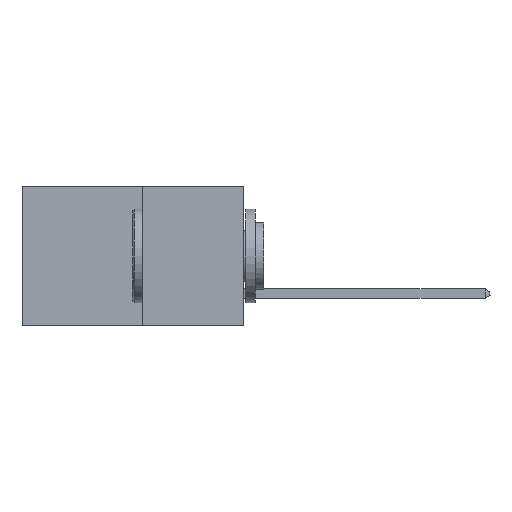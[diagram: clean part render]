
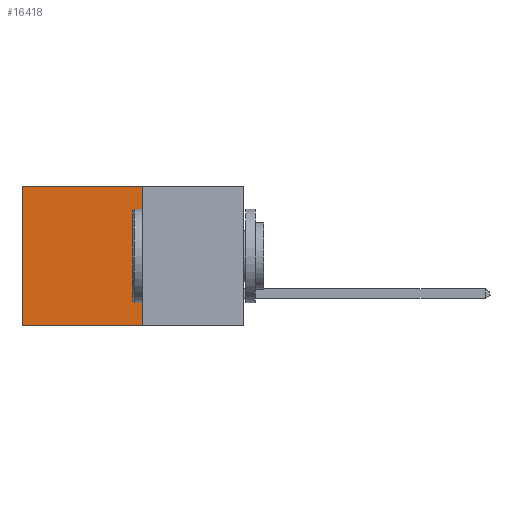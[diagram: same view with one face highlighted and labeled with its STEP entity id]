
A CAD part, left-side view. The second image highlights one B-rep face of the part: STEP entity #16418.
In plain terms, the highlighted planar face has unit normal (-1, 0, 0).
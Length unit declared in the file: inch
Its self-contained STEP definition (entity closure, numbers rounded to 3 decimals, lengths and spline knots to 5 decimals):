
#1302 = EDGE_CURVE ( 'NONE', #14299, #14723, #8624, .T. ) ;
#1588 = VECTOR ( 'NONE', #5379, 39.37008 ) ;
#3808 = LINE ( 'NONE', #8963, #6891 ) ;
#4019 = EDGE_CURVE ( 'NONE', #6749, #14299, #8318, .T. ) ;
#4483 = AXIS2_PLACEMENT_3D ( 'NONE', #4755, #16290, #8631 ) ;
#4755 = CARTESIAN_POINT ( 'NONE',  ( 0.277, 0.27, -0.37 ) ) ;
#4781 = CARTESIAN_POINT ( 'NONE',  ( 0.277, 0.27, -0.37 ) ) ;
#4987 = CARTESIAN_POINT ( 'NONE',  ( 0.277, 0.27, 0. ) ) ;
#5379 = DIRECTION ( 'NONE',  ( 0., 0., -1. ) ) ;
#5942 = VERTEX_POINT ( 'NONE', #13250 ) ;
#6466 = ORIENTED_EDGE ( 'NONE', *, *, #4019, .F. ) ;
#6491 = CARTESIAN_POINT ( 'NONE',  ( 0.277, 0.59, -0.37 ) ) ;
#6749 = VERTEX_POINT ( 'NONE', #11069 ) ;
#6891 = VECTOR ( 'NONE', #16617, 39.37008 ) ;
#7276 = DIRECTION ( 'NONE',  ( 0., 1., 0. ) ) ;
#7335 = PLANE ( 'NONE',  #4483 ) ;
#7648 = FACE_OUTER_BOUND ( 'NONE', #14493, .T. ) ;
#7660 = EDGE_CURVE ( 'NONE', #5942, #14723, #3808, .T. ) ;
#7832 = VECTOR ( 'NONE', #7276, 39.37008 ) ;
#8318 = LINE ( 'NONE', #4781, #1588 ) ;
#8624 = LINE ( 'NONE', #10441, #7832 ) ;
#8631 = DIRECTION ( 'NONE',  ( 0., 0., -1. ) ) ;
#8956 = VECTOR ( 'NONE', #10148, 39.37008 ) ;
#8963 = CARTESIAN_POINT ( 'NONE',  ( 0.277, 0.59, -0.37 ) ) ;
#10148 = DIRECTION ( 'NONE',  ( 0., 1., 0. ) ) ;
#10441 = CARTESIAN_POINT ( 'NONE',  ( 0.277, 0.27, -0.37 ) ) ;
#11069 = CARTESIAN_POINT ( 'NONE',  ( 0.277, 0.27, 0. ) ) ;
#11328 = EDGE_CURVE ( 'NONE', #6749, #5942, #15789, .T. ) ;
#11894 = ORIENTED_EDGE ( 'NONE', *, *, #1302, .F. ) ;
#13238 = CARTESIAN_POINT ( 'NONE',  ( 0.277, 0.27, -0.37 ) ) ;
#13250 = CARTESIAN_POINT ( 'NONE',  ( 0.277, 0.59, 0. ) ) ;
#13385 = ORIENTED_EDGE ( 'NONE', *, *, #7660, .T. ) ;
#14299 = VERTEX_POINT ( 'NONE', #13238 ) ;
#14430 = ORIENTED_EDGE ( 'NONE', *, *, #11328, .T. ) ;
#14493 = EDGE_LOOP ( 'NONE', ( #13385, #11894, #6466, #14430 ) ) ;
#14723 = VERTEX_POINT ( 'NONE', #6491 ) ;
#15789 = LINE ( 'NONE', #4987, #8956 ) ;
#16290 = DIRECTION ( 'NONE',  ( 1., 0., 0. ) ) ;
#16418 = ADVANCED_FACE ( 'NONE', ( #7648 ), #7335, .F. ) ;
#16617 = DIRECTION ( 'NONE',  ( 0., 0., -1. ) ) ;
